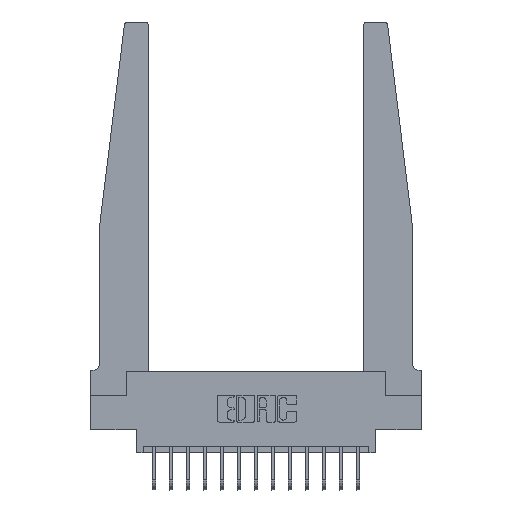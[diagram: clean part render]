
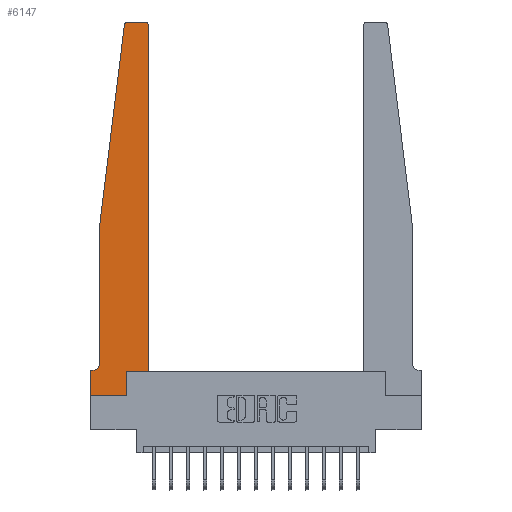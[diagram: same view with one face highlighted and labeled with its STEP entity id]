
A CAD part, top view. The second image highlights one B-rep face of the part: STEP entity #6147.
In plain terms, the highlighted planar face has unit normal (0, 0, 1).
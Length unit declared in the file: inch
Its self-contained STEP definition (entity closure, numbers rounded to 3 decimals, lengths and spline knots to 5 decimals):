
#329 = ORIENTED_EDGE ( 'NONE', *, *, #8467, .T. ) ;
#510 = CARTESIAN_POINT ( 'NONE',  ( 0., 0.1875, 0.37 ) ) ;
#516 = LINE ( 'NONE', #2695, #13620 ) ;
#698 = DIRECTION ( 'NONE',  ( 1., 0., 0. ) ) ;
#775 = VECTOR ( 'NONE', #2676, 39.37008 ) ;
#853 = DIRECTION ( 'NONE',  ( 0., 0., -1. ) ) ;
#1012 = ORIENTED_EDGE ( 'NONE', *, *, #3747, .T. ) ;
#1041 = AXIS2_PLACEMENT_3D ( 'NONE', #12308, #4523, #13603 ) ;
#1069 = LINE ( 'NONE', #1326, #13347 ) ;
#1073 = CARTESIAN_POINT ( 'NONE',  ( 0.24675, 2.72367, 0.37 ) ) ;
#1265 = DIRECTION ( 'NONE',  ( -1., 0., 0. ) ) ;
#1324 = DIRECTION ( 'NONE',  ( -1., 0., 0. ) ) ;
#1326 = CARTESIAN_POINT ( 'NONE',  ( 0.065, 0.1875, 0.37 ) ) ;
#1551 = VERTEX_POINT ( 'NONE', #8663 ) ;
#1916 = ORIENTED_EDGE ( 'NONE', *, *, #8049, .T. ) ;
#2152 = CARTESIAN_POINT ( 'NONE',  ( 0.015, 0.1875, 0.37 ) ) ;
#2278 = AXIS2_PLACEMENT_3D ( 'NONE', #6554, #15599, #7846 ) ;
#2356 = VERTEX_POINT ( 'NONE', #1073 ) ;
#2676 = DIRECTION ( 'NONE',  ( 1., 0., 0. ) ) ;
#2695 = CARTESIAN_POINT ( 'NONE',  ( 0.065, 1.25, 0.37 ) ) ;
#2976 = VERTEX_POINT ( 'NONE', #7699 ) ;
#3032 = CARTESIAN_POINT ( 'NONE',  ( 0.2605, 0.18, 0.37 ) ) ;
#3294 = CARTESIAN_POINT ( 'NONE',  ( 0.2605, 0.18, 0.37 ) ) ;
#3608 = VECTOR ( 'NONE', #1324, 39.37008 ) ;
#3747 = EDGE_CURVE ( 'NONE', #13893, #2356, #12259, .T. ) ;
#4273 = ORIENTED_EDGE ( 'NONE', *, *, #11022, .T. ) ;
#4321 = LINE ( 'NONE', #9207, #775 ) ;
#4523 = DIRECTION ( 'NONE',  ( 0., 0., 1. ) ) ;
#4870 = CARTESIAN_POINT ( 'NONE',  ( 0.2605, 0., 0.37 ) ) ;
#5094 = LINE ( 'NONE', #3032, #14643 ) ;
#5301 = EDGE_CURVE ( 'NONE', #7884, #1551, #516, .T. ) ;
#5364 = DIRECTION ( 'NONE',  ( 0., -1., 0. ) ) ;
#5481 = EDGE_CURVE ( 'NONE', #13488, #15227, #5094, .T. ) ;
#5854 = EDGE_CURVE ( 'NONE', #13999, #2976, #10171, .T. ) ;
#5894 = ORIENTED_EDGE ( 'NONE', *, *, #5481, .T. ) ;
#5989 = ORIENTED_EDGE ( 'NONE', *, *, #15261, .T. ) ;
#6147 = ADVANCED_FACE ( 'NONE', ( #12179 ), #16162, .T. ) ;
#6178 = ORIENTED_EDGE ( 'NONE', *, *, #5301, .T. ) ;
#6331 = EDGE_CURVE ( 'NONE', #2976, #13893, #16227, .T. ) ;
#6554 = CARTESIAN_POINT ( 'NONE',  ( 0.395, 2.72, 0.37 ) ) ;
#6615 = EDGE_CURVE ( 'NONE', #14917, #13488, #9974, .T. ) ;
#6641 = VERTEX_POINT ( 'NONE', #510 ) ;
#6731 = LINE ( 'NONE', #14013, #13181 ) ;
#7547 = DIRECTION ( 'NONE',  ( 0., -1., 0. ) ) ;
#7611 = VECTOR ( 'NONE', #16760, 39.37008 ) ;
#7674 = CIRCLE ( 'NONE', #15740, 0.05 ) ;
#7699 = CARTESIAN_POINT ( 'NONE',  ( 0.395, 2.75, 0.37 ) ) ;
#7828 = LINE ( 'NONE', #12293, #14321 ) ;
#7846 = DIRECTION ( 'NONE',  ( 1., 0., 0. ) ) ;
#7884 = VERTEX_POINT ( 'NONE', #11406 ) ;
#7973 = CARTESIAN_POINT ( 'NONE',  ( 0.25, 2.75, 0.37 ) ) ;
#8049 = EDGE_CURVE ( 'NONE', #12842, #6641, #1069, .T. ) ;
#8256 = CARTESIAN_POINT ( 'NONE',  ( 0.425, 0.18, 0.37 ) ) ;
#8467 = EDGE_CURVE ( 'NONE', #1551, #12842, #7674, .T. ) ;
#8590 = DIRECTION ( 'NONE',  ( 0., 0., 1. ) ) ;
#8663 = CARTESIAN_POINT ( 'NONE',  ( 0.065, 0.2375, 0.37 ) ) ;
#8750 = CARTESIAN_POINT ( 'NONE',  ( 0.015, 0.2375, 0.37 ) ) ;
#9207 = CARTESIAN_POINT ( 'NONE',  ( 0.425, 0.18, 0.37 ) ) ;
#9743 = CARTESIAN_POINT ( 'NONE',  ( 0.27653, 2.75, 0.37 ) ) ;
#9775 = DIRECTION ( 'NONE',  ( 1., 0., 0. ) ) ;
#9974 = LINE ( 'NONE', #16222, #12595 ) ;
#10052 = DIRECTION ( 'NONE',  ( -1., 0., 0. ) ) ;
#10171 = CIRCLE ( 'NONE', #2278, 0.03 ) ;
#10246 = CARTESIAN_POINT ( 'NONE',  ( 0.065, 1.25, 0.37 ) ) ;
#10784 = EDGE_CURVE ( 'NONE', #12645, #13999, #7828, .T. ) ;
#11022 = EDGE_CURVE ( 'NONE', #2356, #7884, #11447, .T. ) ;
#11363 = ORIENTED_EDGE ( 'NONE', *, *, #6331, .T. ) ;
#11406 = CARTESIAN_POINT ( 'NONE',  ( 0.065, 1.25, 0.37 ) ) ;
#11447 = LINE ( 'NONE', #10246, #7611 ) ;
#11670 = ORIENTED_EDGE ( 'NONE', *, *, #11710, .T. ) ;
#11710 = EDGE_CURVE ( 'NONE', #15227, #12645, #4321, .T. ) ;
#11825 = EDGE_LOOP ( 'NONE', ( #11363, #1012, #4273, #6178, #329, #1916, #5989, #12698, #5894, #11670, #12338, #13030 ) ) ;
#12179 = FACE_OUTER_BOUND ( 'NONE', #11825, .T. ) ;
#12259 = CIRCLE ( 'NONE', #12531, 0.03 ) ;
#12293 = CARTESIAN_POINT ( 'NONE',  ( 0.425, 0.18, 0.37 ) ) ;
#12308 = CARTESIAN_POINT ( 'NONE',  ( 0., 0.1875, 0.37 ) ) ;
#12338 = ORIENTED_EDGE ( 'NONE', *, *, #10784, .T. ) ;
#12531 = AXIS2_PLACEMENT_3D ( 'NONE', #16354, #8590, #698 ) ;
#12595 = VECTOR ( 'NONE', #9775, 39.37008 ) ;
#12645 = VERTEX_POINT ( 'NONE', #8256 ) ;
#12698 = ORIENTED_EDGE ( 'NONE', *, *, #6615, .T. ) ;
#12842 = VERTEX_POINT ( 'NONE', #2152 ) ;
#13030 = ORIENTED_EDGE ( 'NONE', *, *, #5854, .T. ) ;
#13181 = VECTOR ( 'NONE', #7547, 39.37008 ) ;
#13347 = VECTOR ( 'NONE', #1265, 39.37008 ) ;
#13450 = DIRECTION ( 'NONE',  ( 0., 1., 0. ) ) ;
#13488 = VERTEX_POINT ( 'NONE', #4870 ) ;
#13588 = DIRECTION ( 'NONE',  ( 0., 1., 0. ) ) ;
#13603 = DIRECTION ( 'NONE',  ( 1., 0., 0. ) ) ;
#13620 = VECTOR ( 'NONE', #5364, 39.37008 ) ;
#13893 = VERTEX_POINT ( 'NONE', #9743 ) ;
#13999 = VERTEX_POINT ( 'NONE', #16652 ) ;
#14013 = CARTESIAN_POINT ( 'NONE',  ( 0., 0., 0.37 ) ) ;
#14321 = VECTOR ( 'NONE', #13588, 39.37008 ) ;
#14365 = CARTESIAN_POINT ( 'NONE',  ( 0., 0., 0.37 ) ) ;
#14643 = VECTOR ( 'NONE', #13450, 39.37008 ) ;
#14917 = VERTEX_POINT ( 'NONE', #14365 ) ;
#15227 = VERTEX_POINT ( 'NONE', #3294 ) ;
#15261 = EDGE_CURVE ( 'NONE', #6641, #14917, #6731, .T. ) ;
#15599 = DIRECTION ( 'NONE',  ( 0., 0., 1. ) ) ;
#15740 = AXIS2_PLACEMENT_3D ( 'NONE', #8750, #853, #10052 ) ;
#16162 = PLANE ( 'NONE',  #1041 ) ;
#16222 = CARTESIAN_POINT ( 'NONE',  ( 0., 0., 0.37 ) ) ;
#16227 = LINE ( 'NONE', #7973, #3608 ) ;
#16354 = CARTESIAN_POINT ( 'NONE',  ( 0.27653, 2.72, 0.37 ) ) ;
#16652 = CARTESIAN_POINT ( 'NONE',  ( 0.425, 2.72, 0.37 ) ) ;
#16760 = DIRECTION ( 'NONE',  ( -0.122, -0.992, 0. ) ) ;
